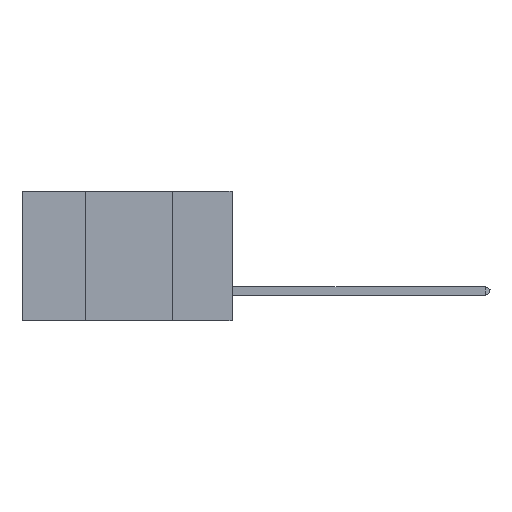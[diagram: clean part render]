
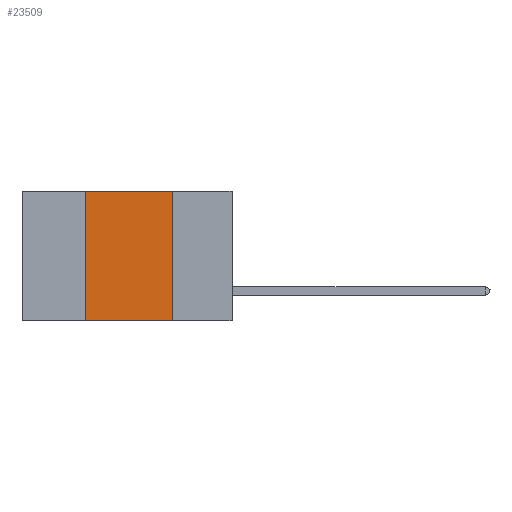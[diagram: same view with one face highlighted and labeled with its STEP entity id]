
A CAD part, left-side view. The second image highlights one B-rep face of the part: STEP entity #23509.
In plain terms, the highlighted planar face has unit normal (-1, 0, 0).
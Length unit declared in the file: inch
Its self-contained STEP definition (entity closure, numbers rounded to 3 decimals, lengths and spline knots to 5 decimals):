
#1617 = EDGE_LOOP ( 'NONE', ( #21613, #32884, #16112, #33006 ) ) ;
#3823 = CARTESIAN_POINT ( 'NONE',  ( 0., 0.42, 0. ) ) ;
#4479 = DIRECTION ( 'NONE',  ( 0., 0., -1. ) ) ;
#5594 = DIRECTION ( 'NONE',  ( 0., 0., -1. ) ) ;
#6863 = VECTOR ( 'NONE', #23404, 39.37008 ) ;
#6979 = EDGE_CURVE ( 'NONE', #16008, #39505, #39882, .T. ) ;
#8026 = CARTESIAN_POINT ( 'NONE',  ( 0., 0.17, 0. ) ) ;
#9745 = CARTESIAN_POINT ( 'NONE',  ( 0., 0.6, -0.37 ) ) ;
#10116 = EDGE_CURVE ( 'NONE', #16008, #25437, #14657, .T. ) ;
#10773 = DIRECTION ( 'NONE',  ( 0., 0., 1. ) ) ;
#11837 = CARTESIAN_POINT ( 'NONE',  ( 0., 0.42, -0.37 ) ) ;
#14657 = LINE ( 'NONE', #3823, #25870 ) ;
#16008 = VERTEX_POINT ( 'NONE', #11837 ) ;
#16112 = ORIENTED_EDGE ( 'NONE', *, *, #10116, .F. ) ;
#17758 = LINE ( 'NONE', #8026, #39562 ) ;
#18064 = AXIS2_PLACEMENT_3D ( 'NONE', #18515, #21246, #5594 ) ;
#18515 = CARTESIAN_POINT ( 'NONE',  ( 0., 0.6, 0. ) ) ;
#18649 = CARTESIAN_POINT ( 'NONE',  ( 0., 0.17, 0. ) ) ;
#21094 = EDGE_CURVE ( 'NONE', #25437, #23572, #34790, .T. ) ;
#21246 = DIRECTION ( 'NONE',  ( 1., 0., 0. ) ) ;
#21247 = FACE_OUTER_BOUND ( 'NONE', #1617, .T. ) ;
#21613 = ORIENTED_EDGE ( 'NONE', *, *, #32666, .F. ) ;
#21702 = VECTOR ( 'NONE', #26547, 39.37008 ) ;
#21990 = CARTESIAN_POINT ( 'NONE',  ( 0., 0.42, 0. ) ) ;
#23404 = DIRECTION ( 'NONE',  ( 0., -1., 0. ) ) ;
#23509 = ADVANCED_FACE ( 'NONE', ( #21247 ), #34220, .F. ) ;
#23550 = CARTESIAN_POINT ( 'NONE',  ( 0., 0.6, 0. ) ) ;
#23572 = VERTEX_POINT ( 'NONE', #18649 ) ;
#25437 = VERTEX_POINT ( 'NONE', #21990 ) ;
#25870 = VECTOR ( 'NONE', #10773, 39.37008 ) ;
#26547 = DIRECTION ( 'NONE',  ( 0., -1., 0. ) ) ;
#32510 = CARTESIAN_POINT ( 'NONE',  ( 0., 0.17, -0.37 ) ) ;
#32666 = EDGE_CURVE ( 'NONE', #23572, #39505, #17758, .T. ) ;
#32884 = ORIENTED_EDGE ( 'NONE', *, *, #21094, .F. ) ;
#33006 = ORIENTED_EDGE ( 'NONE', *, *, #6979, .T. ) ;
#34220 = PLANE ( 'NONE',  #18064 ) ;
#34790 = LINE ( 'NONE', #23550, #21702 ) ;
#39505 = VERTEX_POINT ( 'NONE', #32510 ) ;
#39562 = VECTOR ( 'NONE', #4479, 39.37008 ) ;
#39882 = LINE ( 'NONE', #9745, #6863 ) ;
